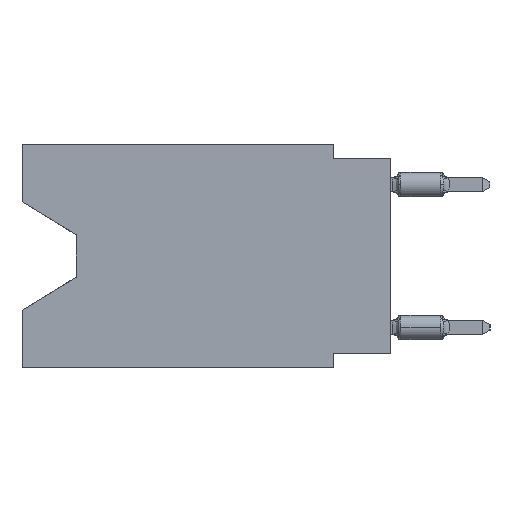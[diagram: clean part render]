
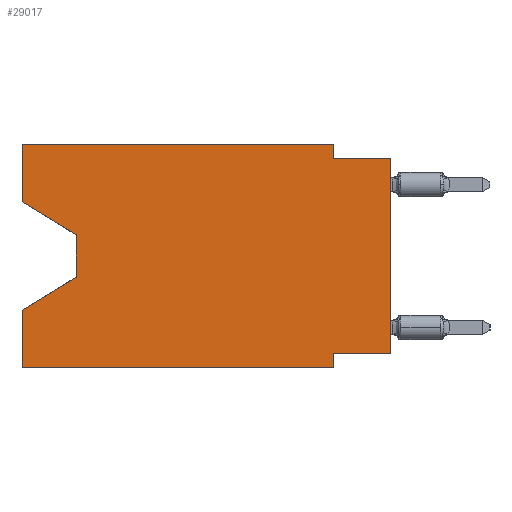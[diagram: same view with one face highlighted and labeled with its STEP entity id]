
A CAD part, left-side view. The second image highlights one B-rep face of the part: STEP entity #29017.
In plain terms, the highlighted planar face has unit normal (-1, 0, 0).
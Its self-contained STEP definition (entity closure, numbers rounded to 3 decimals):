
#835 = DIRECTION ( 'NONE',  ( 0., -1., 0. ) ) ;
#1082 = FACE_OUTER_BOUND ( 'NONE', #27798, .T. ) ;
#2688 = ORIENTED_EDGE ( 'NONE', *, *, #11062, .T. ) ;
#2854 = VERTEX_POINT ( 'NONE', #28608 ) ;
#3218 = VECTOR ( 'NONE', #835, 1000. ) ;
#3376 = CARTESIAN_POINT ( 'NONE',  ( 0., 0., -0.635 ) ) ;
#4266 = VECTOR ( 'NONE', #32311, 1000. ) ;
#4490 = CARTESIAN_POINT ( 'NONE',  ( 0., 13.97, -4.013 ) ) ;
#4501 = AXIS2_PLACEMENT_3D ( 'NONE', #11995, #19529, #8776 ) ;
#6243 = VERTEX_POINT ( 'NONE', #7391 ) ;
#6767 = CARTESIAN_POINT ( 'NONE',  ( 0., 16.383, 0. ) ) ;
#7391 = CARTESIAN_POINT ( 'NONE',  ( 0., 16.383, -7.36 ) ) ;
#7409 = CARTESIAN_POINT ( 'NONE',  ( 0., 13.97, -5.893 ) ) ;
#8374 = ORIENTED_EDGE ( 'NONE', *, *, #19341, .F. ) ;
#8554 = CARTESIAN_POINT ( 'NONE',  ( 0., 0., 0. ) ) ;
#8749 = CARTESIAN_POINT ( 'NONE',  ( 0., 16.383, -9.906 ) ) ;
#8776 = DIRECTION ( 'NONE',  ( 0., 0., -1. ) ) ;
#9103 = DIRECTION ( 'NONE',  ( 0., 0., -1. ) ) ;
#9127 = EDGE_CURVE ( 'NONE', #16212, #13696, #20960, .T. ) ;
#9896 = VERTEX_POINT ( 'NONE', #12790 ) ;
#10422 = LINE ( 'NONE', #7409, #28989 ) ;
#10508 = ORIENTED_EDGE ( 'NONE', *, *, #22334, .F. ) ;
#10660 = CARTESIAN_POINT ( 'NONE',  ( 0., 16.383, 0. ) ) ;
#11062 = EDGE_CURVE ( 'NONE', #25640, #22202, #13299, .T. ) ;
#11093 = VECTOR ( 'NONE', #34263, 1000. ) ;
#11221 = DIRECTION ( 'NONE',  ( 0., 0., 1. ) ) ;
#11560 = LINE ( 'NONE', #8554, #34484 ) ;
#11965 = EDGE_CURVE ( 'NONE', #22202, #17192, #23785, .T. ) ;
#11995 = CARTESIAN_POINT ( 'NONE',  ( 0., 16.383, 0. ) ) ;
#12302 = CARTESIAN_POINT ( 'NONE',  ( 0., 2.54, -9.906 ) ) ;
#12368 = VECTOR ( 'NONE', #31415, 1000. ) ;
#12401 = LINE ( 'NONE', #26395, #11093 ) ;
#12467 = VECTOR ( 'NONE', #22975, 1000. ) ;
#12648 = DIRECTION ( 'NONE',  ( 0., 0., 1. ) ) ;
#12670 = VERTEX_POINT ( 'NONE', #31026 ) ;
#12790 = CARTESIAN_POINT ( 'NONE',  ( 0., 2.54, 0. ) ) ;
#12822 = EDGE_CURVE ( 'NONE', #17192, #6243, #10422, .T. ) ;
#12825 = CARTESIAN_POINT ( 'NONE',  ( 0., 16.383, 0. ) ) ;
#12929 = LINE ( 'NONE', #34603, #12368 ) ;
#13188 = VERTEX_POINT ( 'NONE', #34755 ) ;
#13299 = LINE ( 'NONE', #24096, #4266 ) ;
#13589 = VECTOR ( 'NONE', #12648, 1000. ) ;
#13696 = VERTEX_POINT ( 'NONE', #24784 ) ;
#13739 = ORIENTED_EDGE ( 'NONE', *, *, #33405, .F. ) ;
#14362 = ORIENTED_EDGE ( 'NONE', *, *, #26529, .F. ) ;
#15500 = LINE ( 'NONE', #10660, #17310 ) ;
#15720 = VERTEX_POINT ( 'NONE', #8749 ) ;
#16212 = VERTEX_POINT ( 'NONE', #26095 ) ;
#16305 = VECTOR ( 'NONE', #18572, 1000. ) ;
#16782 = DIRECTION ( 'NONE',  ( 0., -1., 0. ) ) ;
#17192 = VERTEX_POINT ( 'NONE', #21470 ) ;
#17310 = VECTOR ( 'NONE', #29679, 1000. ) ;
#18246 = ORIENTED_EDGE ( 'NONE', *, *, #28559, .F. ) ;
#18572 = DIRECTION ( 'NONE',  ( 0., 0., -1. ) ) ;
#18994 = CARTESIAN_POINT ( 'NONE',  ( 0., 16.383, -2.546 ) ) ;
#19341 = EDGE_CURVE ( 'NONE', #9896, #16212, #12401, .T. ) ;
#19529 = DIRECTION ( 'NONE',  ( 1., 0., 0. ) ) ;
#19565 = CARTESIAN_POINT ( 'NONE',  ( 0., 0., -9.271 ) ) ;
#19806 = ORIENTED_EDGE ( 'NONE', *, *, #12822, .T. ) ;
#19923 = VECTOR ( 'NONE', #16782, 1000. ) ;
#20096 = LINE ( 'NONE', #19565, #12467 ) ;
#20960 = LINE ( 'NONE', #3376, #19923 ) ;
#21350 = CARTESIAN_POINT ( 'NONE',  ( 0., 16.383, 0. ) ) ;
#21470 = CARTESIAN_POINT ( 'NONE',  ( 0., 13.97, -5.893 ) ) ;
#22202 = VERTEX_POINT ( 'NONE', #4490 ) ;
#22334 = EDGE_CURVE ( 'NONE', #13188, #12670, #23065, .T. ) ;
#22975 = DIRECTION ( 'NONE',  ( 0., 1., 0. ) ) ;
#23065 = LINE ( 'NONE', #12302, #24712 ) ;
#23230 = EDGE_CURVE ( 'NONE', #2854, #13696, #11560, .T. ) ;
#23431 = ORIENTED_EDGE ( 'NONE', *, *, #9127, .F. ) ;
#23519 = EDGE_CURVE ( 'NONE', #25640, #28781, #15500, .T. ) ;
#23785 = LINE ( 'NONE', #24486, #16305 ) ;
#23882 = DIRECTION ( 'NONE',  ( 0., 0.855, -0.519 ) ) ;
#24096 = CARTESIAN_POINT ( 'NONE',  ( 0., 16.383, -2.546 ) ) ;
#24486 = CARTESIAN_POINT ( 'NONE',  ( 0., 13.97, -4.013 ) ) ;
#24712 = VECTOR ( 'NONE', #9103, 1000. ) ;
#24784 = CARTESIAN_POINT ( 'NONE',  ( 0., 0., -0.635 ) ) ;
#25579 = LINE ( 'NONE', #6767, #3218 ) ;
#25617 = ORIENTED_EDGE ( 'NONE', *, *, #23519, .F. ) ;
#25640 = VERTEX_POINT ( 'NONE', #18994 ) ;
#26095 = CARTESIAN_POINT ( 'NONE',  ( 0., 2.54, -0.635 ) ) ;
#26300 = LINE ( 'NONE', #12825, #13589 ) ;
#26395 = CARTESIAN_POINT ( 'NONE',  ( 0., 2.54, 0. ) ) ;
#26529 = EDGE_CURVE ( 'NONE', #15720, #6243, #26300, .T. ) ;
#27798 = EDGE_LOOP ( 'NONE', ( #2688, #29825, #19806, #14362, #31748, #10508, #18246, #30026, #23431, #8374, #13739, #25617 ) ) ;
#28559 = EDGE_CURVE ( 'NONE', #2854, #13188, #20096, .T. ) ;
#28608 = CARTESIAN_POINT ( 'NONE',  ( 0., 0., -9.271 ) ) ;
#28781 = VERTEX_POINT ( 'NONE', #21350 ) ;
#28989 = VECTOR ( 'NONE', #23882, 1000. ) ;
#29017 = ADVANCED_FACE ( 'NONE', ( #1082 ), #33154, .F. ) ;
#29679 = DIRECTION ( 'NONE',  ( 0., 0., 1. ) ) ;
#29825 = ORIENTED_EDGE ( 'NONE', *, *, #11965, .T. ) ;
#30026 = ORIENTED_EDGE ( 'NONE', *, *, #23230, .T. ) ;
#31026 = CARTESIAN_POINT ( 'NONE',  ( 0., 2.54, -9.906 ) ) ;
#31415 = DIRECTION ( 'NONE',  ( 0., -1., 0. ) ) ;
#31748 = ORIENTED_EDGE ( 'NONE', *, *, #35133, .T. ) ;
#32311 = DIRECTION ( 'NONE',  ( 0., -0.855, -0.519 ) ) ;
#33154 = PLANE ( 'NONE',  #4501 ) ;
#33405 = EDGE_CURVE ( 'NONE', #28781, #9896, #25579, .T. ) ;
#34263 = DIRECTION ( 'NONE',  ( 0., 0., -1. ) ) ;
#34484 = VECTOR ( 'NONE', #11221, 1000. ) ;
#34603 = CARTESIAN_POINT ( 'NONE',  ( 0., 16.383, -9.906 ) ) ;
#34755 = CARTESIAN_POINT ( 'NONE',  ( 0., 2.54, -9.271 ) ) ;
#35133 = EDGE_CURVE ( 'NONE', #15720, #12670, #12929, .T. ) ;
